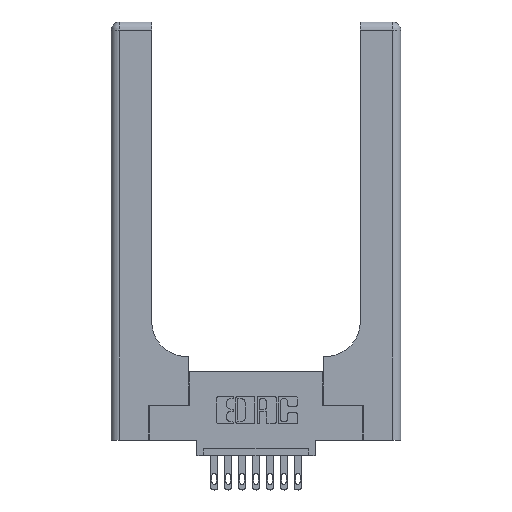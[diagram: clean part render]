
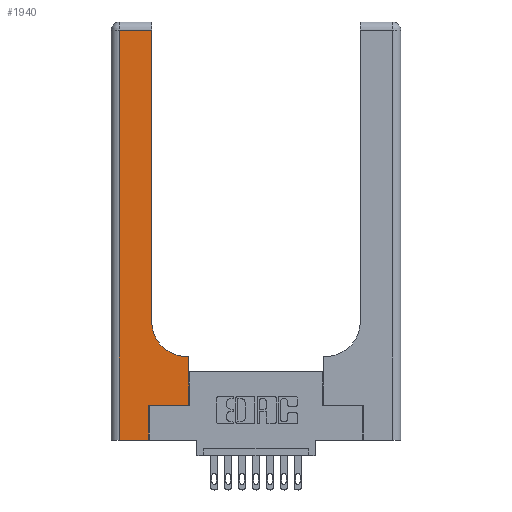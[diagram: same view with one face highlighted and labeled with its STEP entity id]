
A CAD part, top view. The second image highlights one B-rep face of the part: STEP entity #1940.
In plain terms, the highlighted planar face has unit normal (0, 0, 1).
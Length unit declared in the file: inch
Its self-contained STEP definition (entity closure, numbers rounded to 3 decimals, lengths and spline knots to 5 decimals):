
#363 = EDGE_CURVE ( 'NONE', #10638, #14850, #5817, .T. ) ;
#582 = DIRECTION ( 'NONE',  ( 1., 0., 0. ) ) ;
#1185 = LINE ( 'NONE', #8725, #12614 ) ;
#1248 = DIRECTION ( 'NONE',  ( -1., 0., 0. ) ) ;
#1425 = CARTESIAN_POINT ( 'NONE',  ( 0., 2.94, 0.37 ) ) ;
#1581 = ORIENTED_EDGE ( 'NONE', *, *, #5644, .T. ) ;
#1940 = ADVANCED_FACE ( 'NONE', ( #10945 ), #15186, .F. ) ;
#2099 = EDGE_CURVE ( 'NONE', #7872, #12583, #7399, .T. ) ;
#2343 = DIRECTION ( 'NONE',  ( 0., 0., -1. ) ) ;
#2433 = ORIENTED_EDGE ( 'NONE', *, *, #2099, .T. ) ;
#2527 = DIRECTION ( 'NONE',  ( -1., 0., 0. ) ) ;
#2535 = CARTESIAN_POINT ( 'NONE',  ( 0.269, 0., 0.37 ) ) ;
#2937 = EDGE_CURVE ( 'NONE', #14850, #7872, #3536, .T. ) ;
#3536 = LINE ( 'NONE', #14699, #4455 ) ;
#3692 = CARTESIAN_POINT ( 'NONE',  ( 0.2915, 0.6, 0.37 ) ) ;
#3833 = CIRCLE ( 'NONE', #9887, 0.25 ) ;
#3896 = CARTESIAN_POINT ( 'NONE',  ( 0.5585, 0.25, 0.37 ) ) ;
#4174 = CARTESIAN_POINT ( 'NONE',  ( 0.5415, 0.6, 0.37 ) ) ;
#4403 = VECTOR ( 'NONE', #2527, 39.37008 ) ;
#4455 = VECTOR ( 'NONE', #5597, 39.37008 ) ;
#4518 = VERTEX_POINT ( 'NONE', #12607 ) ;
#5201 = CARTESIAN_POINT ( 'NONE',  ( 0.5585, 0.25, 0.37 ) ) ;
#5254 = DIRECTION ( 'NONE',  ( 0., 1., 0. ) ) ;
#5597 = DIRECTION ( 'NONE',  ( 1., 0., 0. ) ) ;
#5644 = EDGE_CURVE ( 'NONE', #14596, #4518, #15242, .T. ) ;
#5767 = VECTOR ( 'NONE', #5254, 39.37008 ) ;
#5817 = LINE ( 'NONE', #14897, #10790 ) ;
#6020 = DIRECTION ( 'NONE',  ( 0., 0., -1. ) ) ;
#6053 = LINE ( 'NONE', #3692, #4403 ) ;
#6131 = VECTOR ( 'NONE', #14467, 39.37008 ) ;
#7106 = CARTESIAN_POINT ( 'NONE',  ( 0.2915, 3., 0.37 ) ) ;
#7157 = AXIS2_PLACEMENT_3D ( 'NONE', #11809, #2343, #1248 ) ;
#7232 = EDGE_LOOP ( 'NONE', ( #13809, #8537, #1581, #13653, #8654, #8196, #2433, #14775, #9976 ) ) ;
#7291 = DIRECTION ( 'NONE',  ( -1., 0., 0. ) ) ;
#7399 = LINE ( 'NONE', #5201, #5767 ) ;
#7823 = DIRECTION ( 'NONE',  ( 0., 1., 0. ) ) ;
#7872 = VERTEX_POINT ( 'NONE', #3896 ) ;
#8196 = ORIENTED_EDGE ( 'NONE', *, *, #2937, .T. ) ;
#8197 = VERTEX_POINT ( 'NONE', #4174 ) ;
#8279 = VERTEX_POINT ( 'NONE', #12840 ) ;
#8537 = ORIENTED_EDGE ( 'NONE', *, *, #11202, .T. ) ;
#8654 = ORIENTED_EDGE ( 'NONE', *, *, #363, .T. ) ;
#8725 = CARTESIAN_POINT ( 'NONE',  ( 0., 0., 0.37 ) ) ;
#9010 = EDGE_CURVE ( 'NONE', #12583, #8197, #6053, .T. ) ;
#9561 = DIRECTION ( 'NONE',  ( 1., 0., 0. ) ) ;
#9608 = EDGE_CURVE ( 'NONE', #8197, #8279, #3833, .T. ) ;
#9887 = AXIS2_PLACEMENT_3D ( 'NONE', #14127, #6020, #9561 ) ;
#9976 = ORIENTED_EDGE ( 'NONE', *, *, #9608, .T. ) ;
#10203 = VERTEX_POINT ( 'NONE', #11886 ) ;
#10638 = VERTEX_POINT ( 'NONE', #2535 ) ;
#10790 = VECTOR ( 'NONE', #7823, 39.37008 ) ;
#10945 = FACE_OUTER_BOUND ( 'NONE', #7232, .T. ) ;
#11202 = EDGE_CURVE ( 'NONE', #10203, #14596, #12081, .T. ) ;
#11204 = CARTESIAN_POINT ( 'NONE',  ( 0.5585, 0.6, 0.37 ) ) ;
#11536 = CARTESIAN_POINT ( 'NONE',  ( 0.06, 2.94, 0.37 ) ) ;
#11809 = CARTESIAN_POINT ( 'NONE',  ( 0., 3., 0.37 ) ) ;
#11886 = CARTESIAN_POINT ( 'NONE',  ( 0.2915, 2.94, 0.37 ) ) ;
#12075 = EDGE_CURVE ( 'NONE', #4518, #10638, #1185, .T. ) ;
#12081 = LINE ( 'NONE', #1425, #12832 ) ;
#12370 = CARTESIAN_POINT ( 'NONE',  ( 0.06, 3., 0.37 ) ) ;
#12467 = EDGE_CURVE ( 'NONE', #8279, #10203, #14076, .T. ) ;
#12583 = VERTEX_POINT ( 'NONE', #11204 ) ;
#12607 = CARTESIAN_POINT ( 'NONE',  ( 0.06, 0., 0.37 ) ) ;
#12614 = VECTOR ( 'NONE', #582, 39.37008 ) ;
#12832 = VECTOR ( 'NONE', #7291, 39.37008 ) ;
#12840 = CARTESIAN_POINT ( 'NONE',  ( 0.2915, 0.85, 0.37 ) ) ;
#13569 = DIRECTION ( 'NONE',  ( 0., -1., 0. ) ) ;
#13653 = ORIENTED_EDGE ( 'NONE', *, *, #12075, .T. ) ;
#13809 = ORIENTED_EDGE ( 'NONE', *, *, #12467, .T. ) ;
#14076 = LINE ( 'NONE', #7106, #6131 ) ;
#14127 = CARTESIAN_POINT ( 'NONE',  ( 0.5415, 0.85, 0.37 ) ) ;
#14425 = CARTESIAN_POINT ( 'NONE',  ( 0.269, 0.25, 0.37 ) ) ;
#14467 = DIRECTION ( 'NONE',  ( 0., 1., 0. ) ) ;
#14596 = VERTEX_POINT ( 'NONE', #11536 ) ;
#14699 = CARTESIAN_POINT ( 'NONE',  ( 0.269, 0.25, 0.37 ) ) ;
#14775 = ORIENTED_EDGE ( 'NONE', *, *, #9010, .T. ) ;
#14850 = VERTEX_POINT ( 'NONE', #14425 ) ;
#14897 = CARTESIAN_POINT ( 'NONE',  ( 0.269, 0., 0.37 ) ) ;
#15068 = VECTOR ( 'NONE', #13569, 39.37008 ) ;
#15186 = PLANE ( 'NONE',  #7157 ) ;
#15242 = LINE ( 'NONE', #12370, #15068 ) ;
